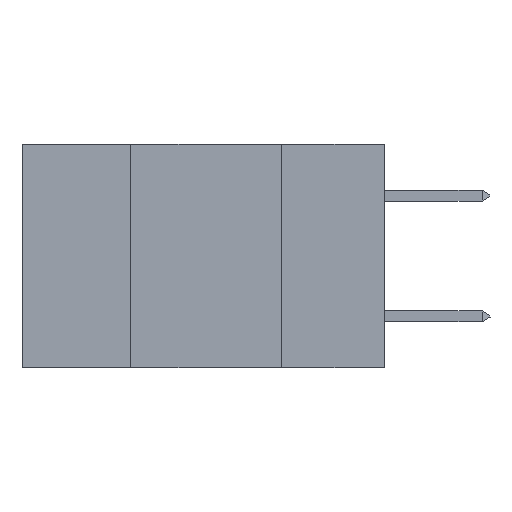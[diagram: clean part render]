
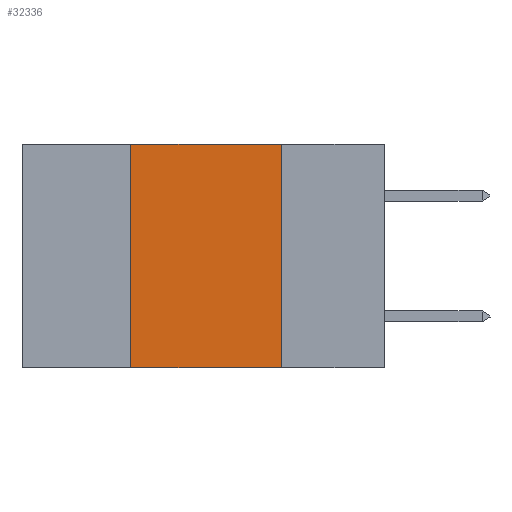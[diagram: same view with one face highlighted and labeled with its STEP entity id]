
A CAD part, left-side view. The second image highlights one B-rep face of the part: STEP entity #32336.
In plain terms, the highlighted planar face has unit normal (-1, 0, 0).
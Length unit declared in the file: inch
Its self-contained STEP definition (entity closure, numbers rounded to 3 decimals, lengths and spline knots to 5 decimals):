
#1400 = EDGE_LOOP ( 'NONE', ( #40577, #17015, #2041, #28117 ) ) ;
#1872 = CARTESIAN_POINT ( 'NONE',  ( 0., 0.42, -0.37 ) ) ;
#2041 = ORIENTED_EDGE ( 'NONE', *, *, #10679, .F. ) ;
#3848 = EDGE_CURVE ( 'NONE', #26881, #3965, #13626, .T. ) ;
#3965 = VERTEX_POINT ( 'NONE', #25146 ) ;
#6345 = EDGE_CURVE ( 'NONE', #22742, #41921, #41684, .T. ) ;
#10679 = EDGE_CURVE ( 'NONE', #22742, #26881, #38411, .T. ) ;
#13280 = VECTOR ( 'NONE', #40119, 39.37008 ) ;
#13445 = CARTESIAN_POINT ( 'NONE',  ( 0., 0.17, 0. ) ) ;
#13626 = LINE ( 'NONE', #41677, #39031 ) ;
#15514 = CARTESIAN_POINT ( 'NONE',  ( 0., 0.6, -0.37 ) ) ;
#16062 = DIRECTION ( 'NONE',  ( 0., 0., -1. ) ) ;
#16136 = DIRECTION ( 'NONE',  ( 0., 0., 1. ) ) ;
#17015 = ORIENTED_EDGE ( 'NONE', *, *, #3848, .F. ) ;
#17257 = AXIS2_PLACEMENT_3D ( 'NONE', #22569, #28839, #16062 ) ;
#18328 = DIRECTION ( 'NONE',  ( 0., -1., 0. ) ) ;
#19607 = CARTESIAN_POINT ( 'NONE',  ( 0., 0.42, 0. ) ) ;
#20308 = VECTOR ( 'NONE', #16136, 39.37008 ) ;
#22569 = CARTESIAN_POINT ( 'NONE',  ( 0., 0.6, 0. ) ) ;
#22742 = VERTEX_POINT ( 'NONE', #1872 ) ;
#25146 = CARTESIAN_POINT ( 'NONE',  ( 0., 0.17, 0. ) ) ;
#26269 = LINE ( 'NONE', #13445, #13280 ) ;
#26881 = VERTEX_POINT ( 'NONE', #38529 ) ;
#27691 = VECTOR ( 'NONE', #28863, 39.37008 ) ;
#28117 = ORIENTED_EDGE ( 'NONE', *, *, #6345, .T. ) ;
#28839 = DIRECTION ( 'NONE',  ( 1., 0., 0. ) ) ;
#28863 = DIRECTION ( 'NONE',  ( 0., -1., 0. ) ) ;
#32336 = ADVANCED_FACE ( 'NONE', ( #35264 ), #42448, .F. ) ;
#34481 = EDGE_CURVE ( 'NONE', #3965, #41921, #26269, .T. ) ;
#35264 = FACE_OUTER_BOUND ( 'NONE', #1400, .T. ) ;
#38411 = LINE ( 'NONE', #19607, #20308 ) ;
#38529 = CARTESIAN_POINT ( 'NONE',  ( 0., 0.42, 0. ) ) ;
#38634 = CARTESIAN_POINT ( 'NONE',  ( 0., 0.17, -0.37 ) ) ;
#39031 = VECTOR ( 'NONE', #18328, 39.37008 ) ;
#40119 = DIRECTION ( 'NONE',  ( 0., 0., -1. ) ) ;
#40577 = ORIENTED_EDGE ( 'NONE', *, *, #34481, .F. ) ;
#41677 = CARTESIAN_POINT ( 'NONE',  ( 0., 0.6, 0. ) ) ;
#41684 = LINE ( 'NONE', #15514, #27691 ) ;
#41921 = VERTEX_POINT ( 'NONE', #38634 ) ;
#42448 = PLANE ( 'NONE',  #17257 ) ;
